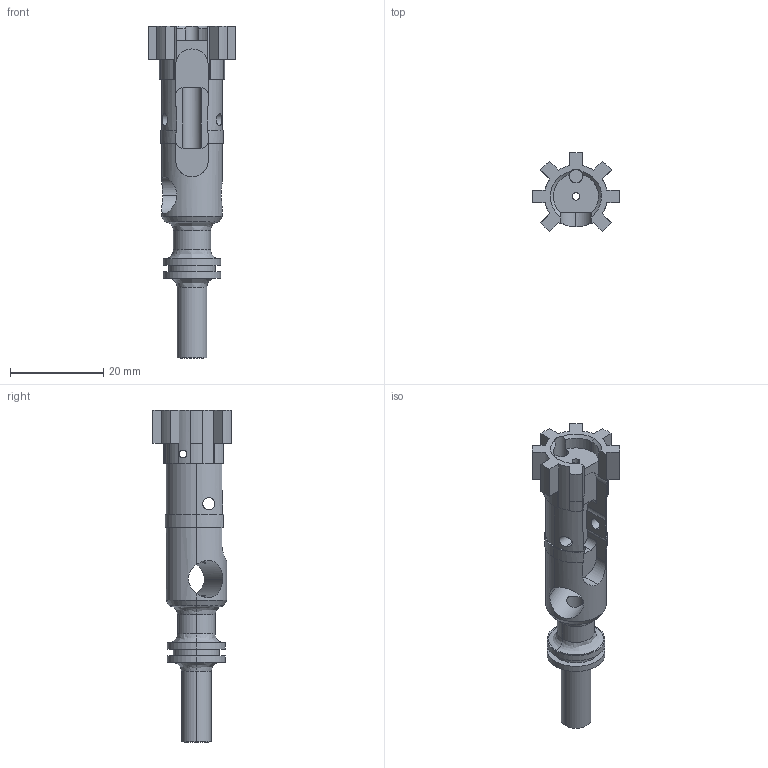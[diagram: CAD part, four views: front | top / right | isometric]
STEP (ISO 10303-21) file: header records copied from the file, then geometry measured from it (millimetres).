
FILE_DESCRIPTION (( 'STEP AP214' ), '1' );
FILE_NAME ('User Library-M4A1 - Bolt Carrier - Assembly_M4A1 - Bolt - Bolt1.STEP', '2013-05-23T12:54:04', ( 'Asher' ), ( '' ), 'SwSTEP 2.0', 'SolidWorks 2013', '' );
FILE_SCHEMA (( 'AUTOMOTIVE_DESIGN' ));
Length unit declared in the file: millimetre
Products named in the file (1): User Library-M4A1 - Bolt Carrier - Assembly_M4A1 - Bolt - Bolt1
Bounding box: 18.78 x 16.9 x 71.07 mm (x, y, z)
Volume: 4759.3 mm3; surface area: 4653 mm2
Topology: 1 solids, 1 shells, 140 faces, 392 edges, 253 vertices
Faces by surface type: cylinder 77, plane 48, cone 9, bspline 6
Entity records: 5486 total; most frequent: CARTESIAN_POINT 1800, ORIENTED_EDGE 784, DIRECTION 758, EDGE_CURVE 392, AXIS2_PLACEMENT_3D 277, VERTEX_POINT 253, LINE 204, VECTOR 204
